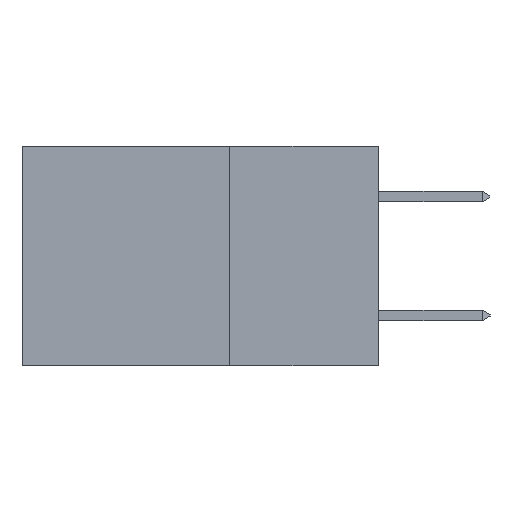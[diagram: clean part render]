
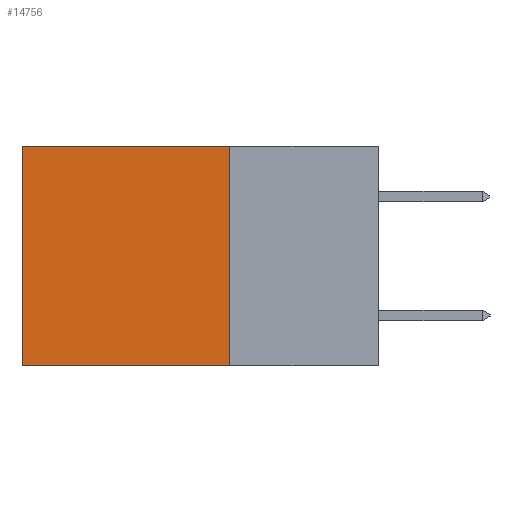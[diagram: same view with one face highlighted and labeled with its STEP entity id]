
A CAD part, left-side view. The second image highlights one B-rep face of the part: STEP entity #14756.
In plain terms, the highlighted planar face has unit normal (-1, 0, 0).
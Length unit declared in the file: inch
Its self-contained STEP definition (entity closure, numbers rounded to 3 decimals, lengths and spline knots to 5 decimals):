
#636 = CARTESIAN_POINT ( 'NONE',  ( 0.2615, 0.25, -0.37 ) ) ;
#885 = DIRECTION ( 'NONE',  ( 0., 0., -1. ) ) ;
#1259 = VECTOR ( 'NONE', #12659, 39.37008 ) ;
#1809 = CARTESIAN_POINT ( 'NONE',  ( 0.2615, 0.25, 0. ) ) ;
#2134 = EDGE_LOOP ( 'NONE', ( #18306, #15648, #15413, #10759 ) ) ;
#4904 = VERTEX_POINT ( 'NONE', #636 ) ;
#6094 = LINE ( 'NONE', #11190, #13365 ) ;
#6506 = VECTOR ( 'NONE', #6898, 39.37008 ) ;
#6823 = CARTESIAN_POINT ( 'NONE',  ( 0.2615, 0.25, -0.37 ) ) ;
#6898 = DIRECTION ( 'NONE',  ( 0., 0., -1. ) ) ;
#7330 = EDGE_CURVE ( 'NONE', #11695, #4904, #10909, .T. ) ;
#7460 = CARTESIAN_POINT ( 'NONE',  ( 0.2615, 0.6, -0.37 ) ) ;
#8115 = FACE_OUTER_BOUND ( 'NONE', #2134, .T. ) ;
#8422 = EDGE_CURVE ( 'NONE', #4904, #14140, #6094, .T. ) ;
#9254 = CARTESIAN_POINT ( 'NONE',  ( 0.2615, 0.25, -0.37 ) ) ;
#9331 = CARTESIAN_POINT ( 'NONE',  ( 0.2615, 0.6, -0.37 ) ) ;
#10030 = AXIS2_PLACEMENT_3D ( 'NONE', #9254, #10907, #885 ) ;
#10180 = LINE ( 'NONE', #9331, #1259 ) ;
#10226 = DIRECTION ( 'NONE',  ( 0., 1., 0. ) ) ;
#10607 = EDGE_CURVE ( 'NONE', #18046, #14140, #10180, .T. ) ;
#10759 = ORIENTED_EDGE ( 'NONE', *, *, #20431, .T. ) ;
#10907 = DIRECTION ( 'NONE',  ( 1., 0., 0. ) ) ;
#10909 = LINE ( 'NONE', #6823, #6506 ) ;
#11190 = CARTESIAN_POINT ( 'NONE',  ( 0.2615, 0.25, -0.37 ) ) ;
#11695 = VERTEX_POINT ( 'NONE', #18623 ) ;
#12659 = DIRECTION ( 'NONE',  ( 0., 0., -1. ) ) ;
#13365 = VECTOR ( 'NONE', #14550, 39.37008 ) ;
#14140 = VERTEX_POINT ( 'NONE', #7460 ) ;
#14550 = DIRECTION ( 'NONE',  ( 0., 1., 0. ) ) ;
#14756 = ADVANCED_FACE ( 'NONE', ( #8115 ), #19305, .F. ) ;
#14769 = CARTESIAN_POINT ( 'NONE',  ( 0.2615, 0.6, 0. ) ) ;
#15326 = VECTOR ( 'NONE', #10226, 39.37008 ) ;
#15413 = ORIENTED_EDGE ( 'NONE', *, *, #7330, .F. ) ;
#15648 = ORIENTED_EDGE ( 'NONE', *, *, #8422, .F. ) ;
#18046 = VERTEX_POINT ( 'NONE', #14769 ) ;
#18306 = ORIENTED_EDGE ( 'NONE', *, *, #10607, .T. ) ;
#18623 = CARTESIAN_POINT ( 'NONE',  ( 0.2615, 0.25, 0. ) ) ;
#19305 = PLANE ( 'NONE',  #10030 ) ;
#19794 = LINE ( 'NONE', #1809, #15326 ) ;
#20431 = EDGE_CURVE ( 'NONE', #11695, #18046, #19794, .T. ) ;
